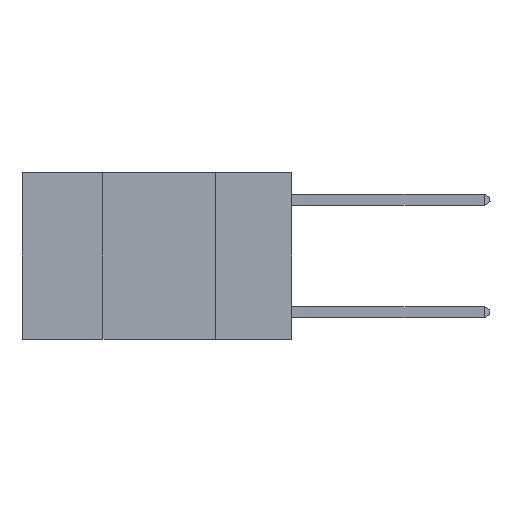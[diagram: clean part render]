
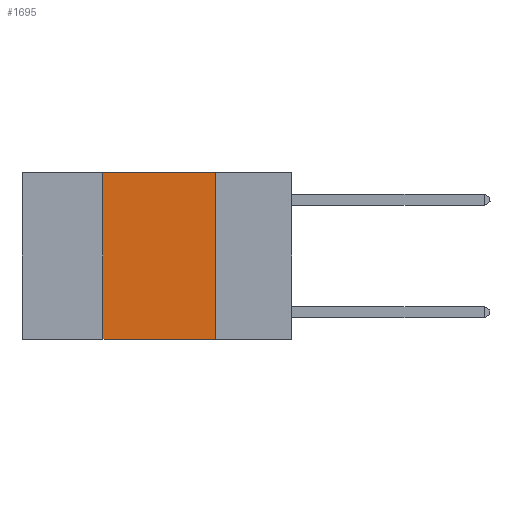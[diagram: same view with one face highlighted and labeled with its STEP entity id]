
A CAD part, left-side view. The second image highlights one B-rep face of the part: STEP entity #1695.
In plain terms, the highlighted planar face has unit normal (-1, 0, 0).
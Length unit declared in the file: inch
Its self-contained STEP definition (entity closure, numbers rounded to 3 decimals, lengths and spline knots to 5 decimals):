
#487 = FACE_OUTER_BOUND ( 'NONE', #8493, .T. ) ;
#888 = VECTOR ( 'NONE', #10073, 39.37008 ) ;
#1264 = ORIENTED_EDGE ( 'NONE', *, *, #5650, .T. ) ;
#1395 = LINE ( 'NONE', #6149, #7572 ) ;
#1488 = DIRECTION ( 'NONE',  ( 0., -1., 0. ) ) ;
#1695 = ADVANCED_FACE ( 'NONE', ( #487 ), #5709, .F. ) ;
#3140 = DIRECTION ( 'NONE',  ( 0., -1., 0. ) ) ;
#3748 = CARTESIAN_POINT ( 'NONE',  ( 0., 0.17, 0. ) ) ;
#3783 = DIRECTION ( 'NONE',  ( 0., 0., 1. ) ) ;
#3814 = LINE ( 'NONE', #8807, #5937 ) ;
#3815 = AXIS2_PLACEMENT_3D ( 'NONE', #7217, #5516, #4859 ) ;
#4475 = CARTESIAN_POINT ( 'NONE',  ( 0., 0.42, 0. ) ) ;
#4587 = ORIENTED_EDGE ( 'NONE', *, *, #6725, .F. ) ;
#4698 = VERTEX_POINT ( 'NONE', #6502 ) ;
#4859 = DIRECTION ( 'NONE',  ( 0., 0., -1. ) ) ;
#5358 = VERTEX_POINT ( 'NONE', #6031 ) ;
#5516 = DIRECTION ( 'NONE',  ( 1., 0., 0. ) ) ;
#5590 = EDGE_CURVE ( 'NONE', #8277, #7556, #8357, .T. ) ;
#5650 = EDGE_CURVE ( 'NONE', #4698, #5358, #3814, .T. ) ;
#5689 = ORIENTED_EDGE ( 'NONE', *, *, #6166, .F. ) ;
#5709 = PLANE ( 'NONE',  #3815 ) ;
#5937 = VECTOR ( 'NONE', #3140, 39.37008 ) ;
#6031 = CARTESIAN_POINT ( 'NONE',  ( 0., 0.17, -0.37 ) ) ;
#6149 = CARTESIAN_POINT ( 'NONE',  ( 0., 0.42, 0. ) ) ;
#6166 = EDGE_CURVE ( 'NONE', #4698, #8277, #1395, .T. ) ;
#6502 = CARTESIAN_POINT ( 'NONE',  ( 0., 0.42, -0.37 ) ) ;
#6725 = EDGE_CURVE ( 'NONE', #7556, #5358, #9496, .T. ) ;
#7123 = CARTESIAN_POINT ( 'NONE',  ( 0., 0.6, 0. ) ) ;
#7217 = CARTESIAN_POINT ( 'NONE',  ( 0., 0.6, 0. ) ) ;
#7474 = ORIENTED_EDGE ( 'NONE', *, *, #5590, .F. ) ;
#7556 = VERTEX_POINT ( 'NONE', #3748 ) ;
#7572 = VECTOR ( 'NONE', #3783, 39.37008 ) ;
#8277 = VERTEX_POINT ( 'NONE', #4475 ) ;
#8357 = LINE ( 'NONE', #7123, #8618 ) ;
#8435 = CARTESIAN_POINT ( 'NONE',  ( 0., 0.17, 0. ) ) ;
#8493 = EDGE_LOOP ( 'NONE', ( #4587, #7474, #5689, #1264 ) ) ;
#8618 = VECTOR ( 'NONE', #1488, 39.37008 ) ;
#8807 = CARTESIAN_POINT ( 'NONE',  ( 0., 0.6, -0.37 ) ) ;
#9496 = LINE ( 'NONE', #8435, #888 ) ;
#10073 = DIRECTION ( 'NONE',  ( 0., 0., -1. ) ) ;
